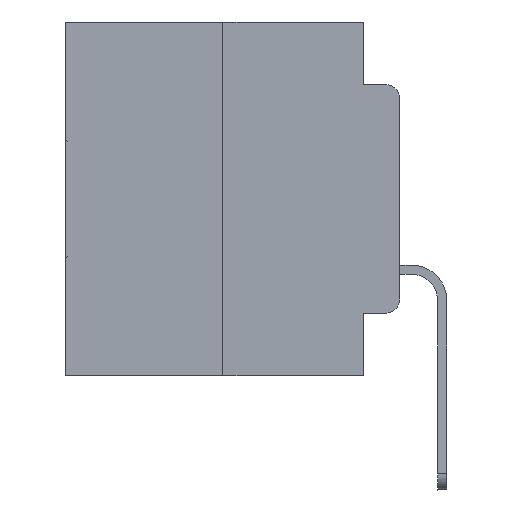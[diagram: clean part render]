
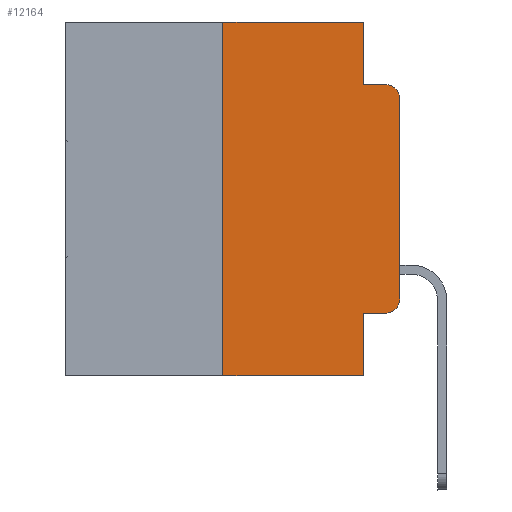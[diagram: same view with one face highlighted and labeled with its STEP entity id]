
A CAD part, left-side view. The second image highlights one B-rep face of the part: STEP entity #12164.
In plain terms, the highlighted planar face has unit normal (-1, 0, 0).
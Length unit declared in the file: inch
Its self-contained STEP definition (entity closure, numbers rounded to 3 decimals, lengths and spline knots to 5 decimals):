
#16 = CARTESIAN_POINT ( 'NONE',  ( 0., 0.051, -0.0885 ) ) ;
#100 = VERTEX_POINT ( 'NONE', #13830 ) ;
#1361 = FACE_OUTER_BOUND ( 'NONE', #7701, .T. ) ;
#1384 = CARTESIAN_POINT ( 'NONE',  ( 0., 0.25, 0. ) ) ;
#2517 = VECTOR ( 'NONE', #24808, 39.37008 ) ;
#2718 = CARTESIAN_POINT ( 'NONE',  ( 0., 0.051, -0.5 ) ) ;
#2720 = DIRECTION ( 'NONE',  ( -1., 0., 0. ) ) ;
#2885 = VECTOR ( 'NONE', #4579, 39.37008 ) ;
#2963 = EDGE_CURVE ( 'NONE', #10536, #21144, #15269, .T. ) ;
#2989 = CARTESIAN_POINT ( 'NONE',  ( 0., 0.02, -0.0885 ) ) ;
#3798 = ORIENTED_EDGE ( 'NONE', *, *, #8333, .F. ) ;
#4153 = ORIENTED_EDGE ( 'NONE', *, *, #16587, .T. ) ;
#4297 = EDGE_CURVE ( 'NONE', #100, #11507, #25980, .T. ) ;
#4579 = DIRECTION ( 'NONE',  ( 0., 0., -1. ) ) ;
#5190 = AXIS2_PLACEMENT_3D ( 'NONE', #13238, #21705, #17401 ) ;
#5356 = CARTESIAN_POINT ( 'NONE',  ( 0., 0., -0.3915 ) ) ;
#5941 = CARTESIAN_POINT ( 'NONE',  ( 0., 0.051, 0. ) ) ;
#6233 = ORIENTED_EDGE ( 'NONE', *, *, #2963, .F. ) ;
#6751 = LINE ( 'NONE', #26193, #2885 ) ;
#7525 = VERTEX_POINT ( 'NONE', #18990 ) ;
#7653 = AXIS2_PLACEMENT_3D ( 'NONE', #22684, #9612, #18372 ) ;
#7701 = EDGE_LOOP ( 'NONE', ( #4153, #15077, #6233, #3798, #21735, #27898, #25153, #24132, #16758, #11451 ) ) ;
#7883 = CARTESIAN_POINT ( 'NONE',  ( 0., 0.051, 0. ) ) ;
#8017 = DIRECTION ( 'NONE',  ( 0., 0., -1. ) ) ;
#8122 = EDGE_CURVE ( 'NONE', #23335, #21144, #25849, .T. ) ;
#8333 = EDGE_CURVE ( 'NONE', #16390, #10536, #20699, .T. ) ;
#8387 = EDGE_CURVE ( 'NONE', #100, #14071, #25318, .T. ) ;
#9612 = DIRECTION ( 'NONE',  ( 1., 0., 0. ) ) ;
#9879 = PLANE ( 'NONE',  #7653 ) ;
#10068 = DIRECTION ( 'NONE',  ( 0., 0., -1. ) ) ;
#10536 = VERTEX_POINT ( 'NONE', #13131 ) ;
#11451 = ORIENTED_EDGE ( 'NONE', *, *, #23700, .T. ) ;
#11507 = VERTEX_POINT ( 'NONE', #2718 ) ;
#12164 = ADVANCED_FACE ( 'NONE', ( #1361 ), #9879, .F. ) ;
#13024 = CARTESIAN_POINT ( 'NONE',  ( 0., 0.473, -0.5 ) ) ;
#13131 = CARTESIAN_POINT ( 'NONE',  ( 0., 0.051, -0.0885 ) ) ;
#13238 = CARTESIAN_POINT ( 'NONE',  ( 0., 0.02, -0.1085 ) ) ;
#13283 = CARTESIAN_POINT ( 'NONE',  ( 0., 0.051, -0.4115 ) ) ;
#13830 = CARTESIAN_POINT ( 'NONE',  ( 0., 0.25, -0.5 ) ) ;
#14071 = VERTEX_POINT ( 'NONE', #15430 ) ;
#14302 = VERTEX_POINT ( 'NONE', #5356 ) ;
#14376 = DIRECTION ( 'NONE',  ( 0., -1., 0. ) ) ;
#14428 = CARTESIAN_POINT ( 'NONE',  ( 0., 0., -0.1085 ) ) ;
#15077 = ORIENTED_EDGE ( 'NONE', *, *, #8122, .T. ) ;
#15269 = LINE ( 'NONE', #16, #26201 ) ;
#15427 = LINE ( 'NONE', #13283, #20966 ) ;
#15430 = CARTESIAN_POINT ( 'NONE',  ( 0., 0.25, 0. ) ) ;
#15679 = VECTOR ( 'NONE', #8017, 39.37008 ) ;
#16390 = VERTEX_POINT ( 'NONE', #5941 ) ;
#16587 = EDGE_CURVE ( 'NONE', #14302, #23335, #20035, .T. ) ;
#16758 = ORIENTED_EDGE ( 'NONE', *, *, #24403, .T. ) ;
#16953 = VERTEX_POINT ( 'NONE', #21993 ) ;
#17401 = DIRECTION ( 'NONE',  ( 0., 0., -1. ) ) ;
#18372 = DIRECTION ( 'NONE',  ( 0., 0., -1. ) ) ;
#18990 = CARTESIAN_POINT ( 'NONE',  ( 0., 0.051, -0.4115 ) ) ;
#19884 = DIRECTION ( 'NONE',  ( 0., -1., 0. ) ) ;
#20035 = LINE ( 'NONE', #24372, #2517 ) ;
#20313 = DIRECTION ( 'NONE',  ( 0., -1., 0. ) ) ;
#20699 = LINE ( 'NONE', #7883, #15679 ) ;
#20836 = CARTESIAN_POINT ( 'NONE',  ( 0., 0.473, 0. ) ) ;
#20939 = VECTOR ( 'NONE', #14376, 39.37008 ) ;
#20966 = VECTOR ( 'NONE', #19884, 39.37008 ) ;
#21069 = EDGE_CURVE ( 'NONE', #7525, #11507, #6751, .T. ) ;
#21109 = LINE ( 'NONE', #20836, #20939 ) ;
#21144 = VERTEX_POINT ( 'NONE', #2989 ) ;
#21705 = DIRECTION ( 'NONE',  ( -1., 0., 0. ) ) ;
#21735 = ORIENTED_EDGE ( 'NONE', *, *, #23837, .F. ) ;
#21993 = CARTESIAN_POINT ( 'NONE',  ( 0., 0.02, -0.4115 ) ) ;
#22440 = CARTESIAN_POINT ( 'NONE',  ( 0., 0.02, -0.3915 ) ) ;
#22684 = CARTESIAN_POINT ( 'NONE',  ( 0., 0.473, 0. ) ) ;
#22788 = CIRCLE ( 'NONE', #24648, 0.02 ) ;
#23335 = VERTEX_POINT ( 'NONE', #14428 ) ;
#23700 = EDGE_CURVE ( 'NONE', #16953, #14302, #22788, .T. ) ;
#23837 = EDGE_CURVE ( 'NONE', #14071, #16390, #21109, .T. ) ;
#24132 = ORIENTED_EDGE ( 'NONE', *, *, #21069, .F. ) ;
#24372 = CARTESIAN_POINT ( 'NONE',  ( 0., 0., 0. ) ) ;
#24403 = EDGE_CURVE ( 'NONE', #7525, #16953, #15427, .T. ) ;
#24648 = AXIS2_PLACEMENT_3D ( 'NONE', #22440, #2720, #10068 ) ;
#24808 = DIRECTION ( 'NONE',  ( 0., 0., 1. ) ) ;
#25153 = ORIENTED_EDGE ( 'NONE', *, *, #4297, .T. ) ;
#25318 = LINE ( 'NONE', #1384, #28122 ) ;
#25587 = DIRECTION ( 'NONE',  ( 0., 0., 1. ) ) ;
#25849 = CIRCLE ( 'NONE', #5190, 0.02 ) ;
#25980 = LINE ( 'NONE', #13024, #28341 ) ;
#26193 = CARTESIAN_POINT ( 'NONE',  ( 0., 0.051, 0. ) ) ;
#26201 = VECTOR ( 'NONE', #28084, 39.37008 ) ;
#27898 = ORIENTED_EDGE ( 'NONE', *, *, #8387, .F. ) ;
#28084 = DIRECTION ( 'NONE',  ( 0., -1., 0. ) ) ;
#28122 = VECTOR ( 'NONE', #25587, 39.37008 ) ;
#28341 = VECTOR ( 'NONE', #20313, 39.37008 ) ;
